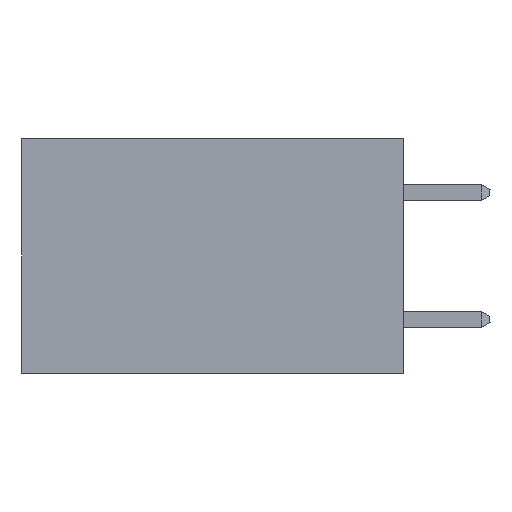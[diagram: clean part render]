
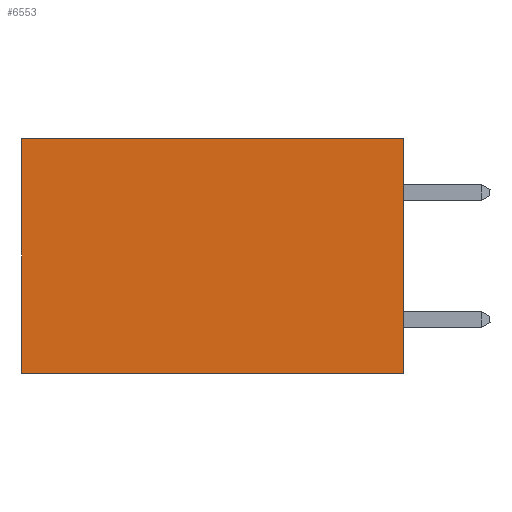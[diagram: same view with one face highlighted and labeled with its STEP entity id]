
A CAD part, left-side view. The second image highlights one B-rep face of the part: STEP entity #6553.
In plain terms, the highlighted planar face has unit normal (-1, 0, 0).
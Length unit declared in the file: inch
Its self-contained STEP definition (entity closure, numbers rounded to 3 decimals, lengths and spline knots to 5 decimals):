
#43 = CARTESIAN_POINT ( 'NONE',  ( 0.2875, 0.6, 0. ) ) ;
#846 = VECTOR ( 'NONE', #4004, 39.37008 ) ;
#1322 = CARTESIAN_POINT ( 'NONE',  ( 0.2875, 0., -0.37 ) ) ;
#2108 = VERTEX_POINT ( 'NONE', #43 ) ;
#3038 = CARTESIAN_POINT ( 'NONE',  ( 0.2875, 0., 0. ) ) ;
#3093 = DIRECTION ( 'NONE',  ( 0., 0., -1. ) ) ;
#3109 = AXIS2_PLACEMENT_3D ( 'NONE', #3038, #12420, #5419 ) ;
#3429 = DIRECTION ( 'NONE',  ( 0., 1., 0. ) ) ;
#3598 = LINE ( 'NONE', #13626, #6347 ) ;
#3841 = LINE ( 'NONE', #12202, #12803 ) ;
#4004 = DIRECTION ( 'NONE',  ( 0., 1., 0. ) ) ;
#5234 = ORIENTED_EDGE ( 'NONE', *, *, #10162, .F. ) ;
#5419 = DIRECTION ( 'NONE',  ( 0., 0., -1. ) ) ;
#5667 = ORIENTED_EDGE ( 'NONE', *, *, #9055, .T. ) ;
#6157 = VERTEX_POINT ( 'NONE', #10611 ) ;
#6347 = VECTOR ( 'NONE', #3093, 39.37008 ) ;
#6553 = ADVANCED_FACE ( 'NONE', ( #6948 ), #13522, .F. ) ;
#6687 = LINE ( 'NONE', #8676, #846 ) ;
#6948 = FACE_OUTER_BOUND ( 'NONE', #12869, .T. ) ;
#6994 = CARTESIAN_POINT ( 'NONE',  ( 0.2875, 0., 0. ) ) ;
#7002 = EDGE_CURVE ( 'NONE', #11804, #14654, #3841, .T. ) ;
#8676 = CARTESIAN_POINT ( 'NONE',  ( 0.2875, 0., -0.37 ) ) ;
#9055 = EDGE_CURVE ( 'NONE', #2108, #6157, #3598, .T. ) ;
#9642 = ORIENTED_EDGE ( 'NONE', *, *, #7002, .F. ) ;
#10162 = EDGE_CURVE ( 'NONE', #14654, #6157, #6687, .T. ) ;
#10611 = CARTESIAN_POINT ( 'NONE',  ( 0.2875, 0.6, -0.37 ) ) ;
#11152 = ORIENTED_EDGE ( 'NONE', *, *, #13745, .T. ) ;
#11804 = VERTEX_POINT ( 'NONE', #6994 ) ;
#12202 = CARTESIAN_POINT ( 'NONE',  ( 0.2875, 0., 0. ) ) ;
#12420 = DIRECTION ( 'NONE',  ( 1., 0., 0. ) ) ;
#12787 = CARTESIAN_POINT ( 'NONE',  ( 0.2875, 0., 0. ) ) ;
#12803 = VECTOR ( 'NONE', #13344, 39.37008 ) ;
#12869 = EDGE_LOOP ( 'NONE', ( #5667, #5234, #9642, #11152 ) ) ;
#13344 = DIRECTION ( 'NONE',  ( 0., 0., -1. ) ) ;
#13522 = PLANE ( 'NONE',  #3109 ) ;
#13626 = CARTESIAN_POINT ( 'NONE',  ( 0.2875, 0.6, 0. ) ) ;
#13745 = EDGE_CURVE ( 'NONE', #11804, #2108, #14964, .T. ) ;
#14604 = VECTOR ( 'NONE', #3429, 39.37008 ) ;
#14654 = VERTEX_POINT ( 'NONE', #1322 ) ;
#14964 = LINE ( 'NONE', #12787, #14604 ) ;
